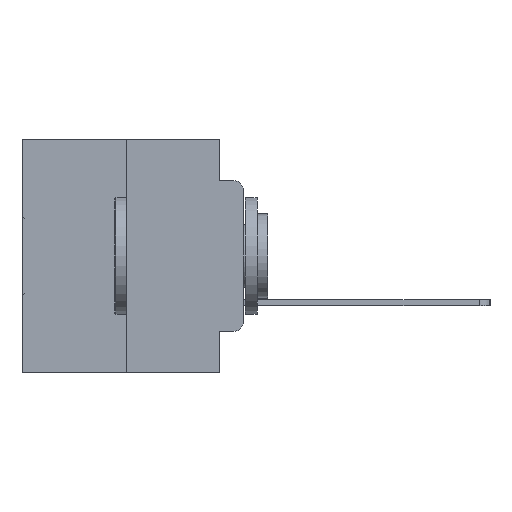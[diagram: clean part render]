
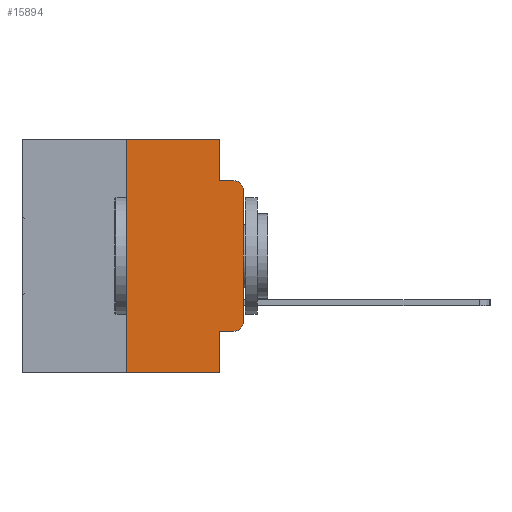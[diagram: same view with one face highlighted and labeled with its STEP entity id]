
A CAD part, left-side view. The second image highlights one B-rep face of the part: STEP entity #15894.
In plain terms, the highlighted planar face has unit normal (-1, 0, 0).
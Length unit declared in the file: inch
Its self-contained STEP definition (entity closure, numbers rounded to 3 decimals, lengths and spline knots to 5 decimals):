
#833 = EDGE_CURVE ( 'NONE', #8328, #27966, #19118, .T. ) ;
#904 = DIRECTION ( 'NONE',  ( 0., 0., -1. ) ) ;
#1299 = VECTOR ( 'NONE', #904, 39.37008 ) ;
#1671 = CIRCLE ( 'NONE', #10097, 0.02 ) ;
#2018 = CARTESIAN_POINT ( 'NONE',  ( 0., 0.473, 0. ) ) ;
#2037 = ORIENTED_EDGE ( 'NONE', *, *, #17206, .T. ) ;
#2307 = EDGE_CURVE ( 'NONE', #8102, #30813, #26320, .T. ) ;
#2489 = EDGE_CURVE ( 'NONE', #26490, #27966, #21930, .T. ) ;
#3068 = DIRECTION ( 'NONE',  ( 0., 0., -1. ) ) ;
#3123 = CARTESIAN_POINT ( 'NONE',  ( 0., 0.02, -0.3915 ) ) ;
#3625 = ORIENTED_EDGE ( 'NONE', *, *, #2489, .T. ) ;
#3735 = LINE ( 'NONE', #10375, #15771 ) ;
#4134 = EDGE_CURVE ( 'NONE', #9440, #26490, #14086, .T. ) ;
#4491 = DIRECTION ( 'NONE',  ( 0., 0., -1. ) ) ;
#5581 = DIRECTION ( 'NONE',  ( 0., 0., -1. ) ) ;
#6331 = VECTOR ( 'NONE', #17100, 39.37008 ) ;
#7327 = CARTESIAN_POINT ( 'NONE',  ( 0., 0.051, -0.0885 ) ) ;
#7394 = VECTOR ( 'NONE', #25804, 39.37008 ) ;
#7672 = CARTESIAN_POINT ( 'NONE',  ( 0., 0.25, -0.5 ) ) ;
#7910 = ORIENTED_EDGE ( 'NONE', *, *, #19238, .F. ) ;
#8102 = VERTEX_POINT ( 'NONE', #7672 ) ;
#8219 = ORIENTED_EDGE ( 'NONE', *, *, #10699, .F. ) ;
#8303 = VECTOR ( 'NONE', #25478, 39.37008 ) ;
#8328 = VERTEX_POINT ( 'NONE', #10942 ) ;
#8776 = VERTEX_POINT ( 'NONE', #24339 ) ;
#8823 = DIRECTION ( 'NONE',  ( 0., -1., 0. ) ) ;
#9033 = CARTESIAN_POINT ( 'NONE',  ( 0., 0.051, 0. ) ) ;
#9131 = CARTESIAN_POINT ( 'NONE',  ( 0., 0.051, -0.4115 ) ) ;
#9440 = VERTEX_POINT ( 'NONE', #26771 ) ;
#9810 = LINE ( 'NONE', #23125, #8303 ) ;
#9971 = DIRECTION ( 'NONE',  ( 0., -1., 0. ) ) ;
#10097 = AXIS2_PLACEMENT_3D ( 'NONE', #3123, #19939, #5581 ) ;
#10327 = VECTOR ( 'NONE', #8823, 39.37008 ) ;
#10375 = CARTESIAN_POINT ( 'NONE',  ( 0., 0.473, 0. ) ) ;
#10699 = EDGE_CURVE ( 'NONE', #8776, #28975, #3735, .T. ) ;
#10942 = CARTESIAN_POINT ( 'NONE',  ( 0., 0.051, -0.0885 ) ) ;
#13121 = ORIENTED_EDGE ( 'NONE', *, *, #27072, .F. ) ;
#13337 = VECTOR ( 'NONE', #30280, 39.37008 ) ;
#13436 = AXIS2_PLACEMENT_3D ( 'NONE', #29113, #17488, #3068 ) ;
#13479 = CARTESIAN_POINT ( 'NONE',  ( 0., 0., 0. ) ) ;
#13518 = LINE ( 'NONE', #28836, #6331 ) ;
#13653 = CARTESIAN_POINT ( 'NONE',  ( 0., 0.051, -0.4115 ) ) ;
#13811 = ORIENTED_EDGE ( 'NONE', *, *, #4134, .T. ) ;
#14086 = LINE ( 'NONE', #13479, #13337 ) ;
#14145 = CARTESIAN_POINT ( 'NONE',  ( 0., 0.473, -0.5 ) ) ;
#15153 = DIRECTION ( 'NONE',  ( 0., -1., 0. ) ) ;
#15219 = ORIENTED_EDGE ( 'NONE', *, *, #15589, .T. ) ;
#15406 = CARTESIAN_POINT ( 'NONE',  ( 0., 0.051, 0. ) ) ;
#15589 = EDGE_CURVE ( 'NONE', #24566, #9440, #1671, .T. ) ;
#15631 = CARTESIAN_POINT ( 'NONE',  ( 0., 0., -0.1085 ) ) ;
#15771 = VECTOR ( 'NONE', #15153, 39.37008 ) ;
#15894 = ADVANCED_FACE ( 'NONE', ( #23734 ), #28118, .F. ) ;
#15977 = EDGE_LOOP ( 'NONE', ( #13811, #3625, #23818, #13121, #8219, #30110, #24963, #7910, #2037, #15219 ) ) ;
#17100 = DIRECTION ( 'NONE',  ( 0., 0., -1. ) ) ;
#17206 = EDGE_CURVE ( 'NONE', #21373, #24566, #23653, .T. ) ;
#17488 = DIRECTION ( 'NONE',  ( -1., 0., 0. ) ) ;
#18367 = VECTOR ( 'NONE', #9971, 39.37008 ) ;
#18893 = DIRECTION ( 'NONE',  ( 1., 0., 0. ) ) ;
#19036 = CARTESIAN_POINT ( 'NONE',  ( 0., 0.02, -0.0885 ) ) ;
#19118 = LINE ( 'NONE', #7327, #18367 ) ;
#19238 = EDGE_CURVE ( 'NONE', #21373, #30813, #13518, .T. ) ;
#19939 = DIRECTION ( 'NONE',  ( -1., 0., 0. ) ) ;
#20510 = LINE ( 'NONE', #15406, #1299 ) ;
#21040 = CARTESIAN_POINT ( 'NONE',  ( 0., 0.051, -0.5 ) ) ;
#21373 = VERTEX_POINT ( 'NONE', #9131 ) ;
#21930 = CIRCLE ( 'NONE', #13436, 0.02 ) ;
#23125 = CARTESIAN_POINT ( 'NONE',  ( 0., 0.25, 0. ) ) ;
#23653 = LINE ( 'NONE', #13653, #10327 ) ;
#23734 = FACE_OUTER_BOUND ( 'NONE', #15977, .T. ) ;
#23818 = ORIENTED_EDGE ( 'NONE', *, *, #833, .F. ) ;
#24101 = CARTESIAN_POINT ( 'NONE',  ( 0., 0.02, -0.4115 ) ) ;
#24339 = CARTESIAN_POINT ( 'NONE',  ( 0., 0.25, 0. ) ) ;
#24566 = VERTEX_POINT ( 'NONE', #24101 ) ;
#24963 = ORIENTED_EDGE ( 'NONE', *, *, #2307, .T. ) ;
#25478 = DIRECTION ( 'NONE',  ( 0., 0., 1. ) ) ;
#25484 = EDGE_CURVE ( 'NONE', #8102, #8776, #9810, .T. ) ;
#25804 = DIRECTION ( 'NONE',  ( 0., -1., 0. ) ) ;
#26320 = LINE ( 'NONE', #14145, #7394 ) ;
#26490 = VERTEX_POINT ( 'NONE', #15631 ) ;
#26771 = CARTESIAN_POINT ( 'NONE',  ( 0., 0., -0.3915 ) ) ;
#27072 = EDGE_CURVE ( 'NONE', #28975, #8328, #20510, .T. ) ;
#27966 = VERTEX_POINT ( 'NONE', #19036 ) ;
#28118 = PLANE ( 'NONE',  #28532 ) ;
#28532 = AXIS2_PLACEMENT_3D ( 'NONE', #2018, #18893, #4491 ) ;
#28836 = CARTESIAN_POINT ( 'NONE',  ( 0., 0.051, 0. ) ) ;
#28975 = VERTEX_POINT ( 'NONE', #9033 ) ;
#29113 = CARTESIAN_POINT ( 'NONE',  ( 0., 0.02, -0.1085 ) ) ;
#30110 = ORIENTED_EDGE ( 'NONE', *, *, #25484, .F. ) ;
#30280 = DIRECTION ( 'NONE',  ( 0., 0., 1. ) ) ;
#30813 = VERTEX_POINT ( 'NONE', #21040 ) ;
